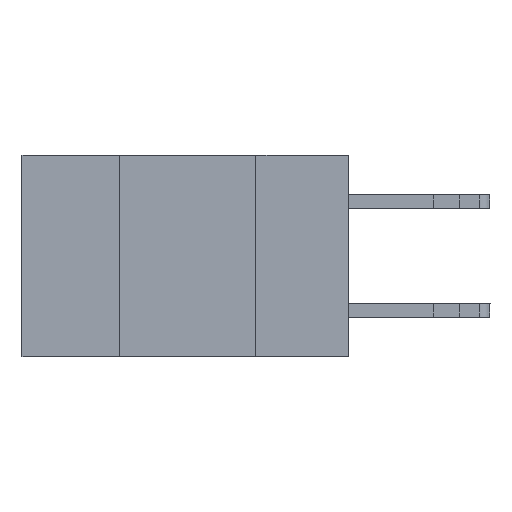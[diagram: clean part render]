
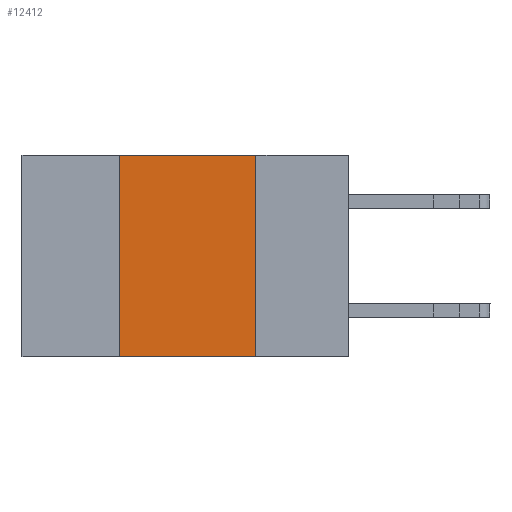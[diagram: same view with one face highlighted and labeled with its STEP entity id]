
A CAD part, left-side view. The second image highlights one B-rep face of the part: STEP entity #12412.
In plain terms, the highlighted planar face has unit normal (-1, 0, 0).
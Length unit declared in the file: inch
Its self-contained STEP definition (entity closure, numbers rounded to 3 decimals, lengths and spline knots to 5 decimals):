
#472 = CARTESIAN_POINT ( 'NONE',  ( 0., 0.6, 0. ) ) ;
#628 = CARTESIAN_POINT ( 'NONE',  ( 0., 0.42, 0. ) ) ;
#1129 = VERTEX_POINT ( 'NONE', #10029 ) ;
#1252 = LINE ( 'NONE', #6374, #5118 ) ;
#1833 = DIRECTION ( 'NONE',  ( 0., 0., -1. ) ) ;
#2211 = CARTESIAN_POINT ( 'NONE',  ( 0., 0.6, -0.37 ) ) ;
#2511 = VECTOR ( 'NONE', #11966, 39.37008 ) ;
#3617 = DIRECTION ( 'NONE',  ( 0., 0., -1. ) ) ;
#3689 = EDGE_LOOP ( 'NONE', ( #15672, #12784, #14808, #10247 ) ) ;
#3815 = EDGE_CURVE ( 'NONE', #15722, #14378, #1252, .T. ) ;
#3825 = AXIS2_PLACEMENT_3D ( 'NONE', #472, #10082, #1833 ) ;
#5051 = DIRECTION ( 'NONE',  ( 0., -1., 0. ) ) ;
#5118 = VECTOR ( 'NONE', #3617, 39.37008 ) ;
#6027 = EDGE_CURVE ( 'NONE', #10120, #15722, #9832, .T. ) ;
#6374 = CARTESIAN_POINT ( 'NONE',  ( 0., 0.17, 0. ) ) ;
#6667 = EDGE_CURVE ( 'NONE', #1129, #10120, #17518, .T. ) ;
#6736 = CARTESIAN_POINT ( 'NONE',  ( 0., 0.17, 0. ) ) ;
#7790 = CARTESIAN_POINT ( 'NONE',  ( 0., 0.6, 0. ) ) ;
#8869 = PLANE ( 'NONE',  #3825 ) ;
#9832 = LINE ( 'NONE', #7790, #2511 ) ;
#10029 = CARTESIAN_POINT ( 'NONE',  ( 0., 0.42, -0.37 ) ) ;
#10082 = DIRECTION ( 'NONE',  ( 1., 0., 0. ) ) ;
#10120 = VERTEX_POINT ( 'NONE', #10942 ) ;
#10247 = ORIENTED_EDGE ( 'NONE', *, *, #11165, .T. ) ;
#10942 = CARTESIAN_POINT ( 'NONE',  ( 0., 0.42, 0. ) ) ;
#11165 = EDGE_CURVE ( 'NONE', #1129, #14378, #16244, .T. ) ;
#11966 = DIRECTION ( 'NONE',  ( 0., -1., 0. ) ) ;
#12412 = ADVANCED_FACE ( 'NONE', ( #14749 ), #8869, .F. ) ;
#12784 = ORIENTED_EDGE ( 'NONE', *, *, #6027, .F. ) ;
#13088 = VECTOR ( 'NONE', #5051, 39.37008 ) ;
#13868 = CARTESIAN_POINT ( 'NONE',  ( 0., 0.17, -0.37 ) ) ;
#14378 = VERTEX_POINT ( 'NONE', #13868 ) ;
#14749 = FACE_OUTER_BOUND ( 'NONE', #3689, .T. ) ;
#14808 = ORIENTED_EDGE ( 'NONE', *, *, #6667, .F. ) ;
#15672 = ORIENTED_EDGE ( 'NONE', *, *, #3815, .F. ) ;
#15680 = DIRECTION ( 'NONE',  ( 0., 0., 1. ) ) ;
#15722 = VERTEX_POINT ( 'NONE', #6736 ) ;
#16244 = LINE ( 'NONE', #2211, #13088 ) ;
#17077 = VECTOR ( 'NONE', #15680, 39.37008 ) ;
#17518 = LINE ( 'NONE', #628, #17077 ) ;
